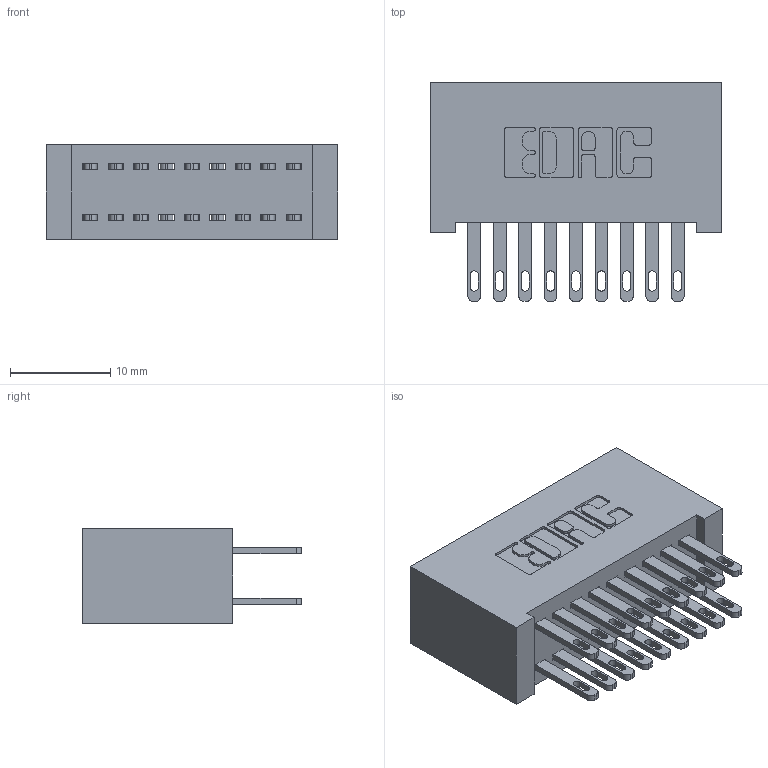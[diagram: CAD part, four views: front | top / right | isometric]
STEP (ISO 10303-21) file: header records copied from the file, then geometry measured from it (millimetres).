
FILE_DESCRIPTION (( 'STEP AP203' ), '1' );
FILE_NAME ('892-018-500-201.STEP', '2020-09-21T13:42:27', ( '' ), ( '' ), 'SwSTEP 2.0', 'SolidWorks 2020', '' );
FILE_SCHEMA (( 'CONFIG_CONTROL_DESIGN' ));
Length unit declared in the file: inch
Products named in the file (3): 892-018-500-201; 345-292-001_345-293-100; 842 Part_Lugless
Assembly tree (19 placements, depth 2):
  892-018-500-201
    842 Part_Lugless
    345-292-001_345-293-100  x18
Bounding box: 29.11 x 21.85 x 9.4 mm (x, y, z)
Volume: 2953.7 mm3; surface area: 4613.3 mm2
Topology: 19 solids, 19 shells, 966 faces, 2921 edges, 1946 vertices
Faces by surface type: plane 602, cylinder 364
Entity records: 9579 total; most frequent: CARTESIAN_POINT 1622, ORIENTED_EDGE 1558, DIRECTION 1439, EDGE_CURVE 779, VECTOR 655, LINE 655, VERTEX_POINT 518, AXIS2_PLACEMENT_3D 392
